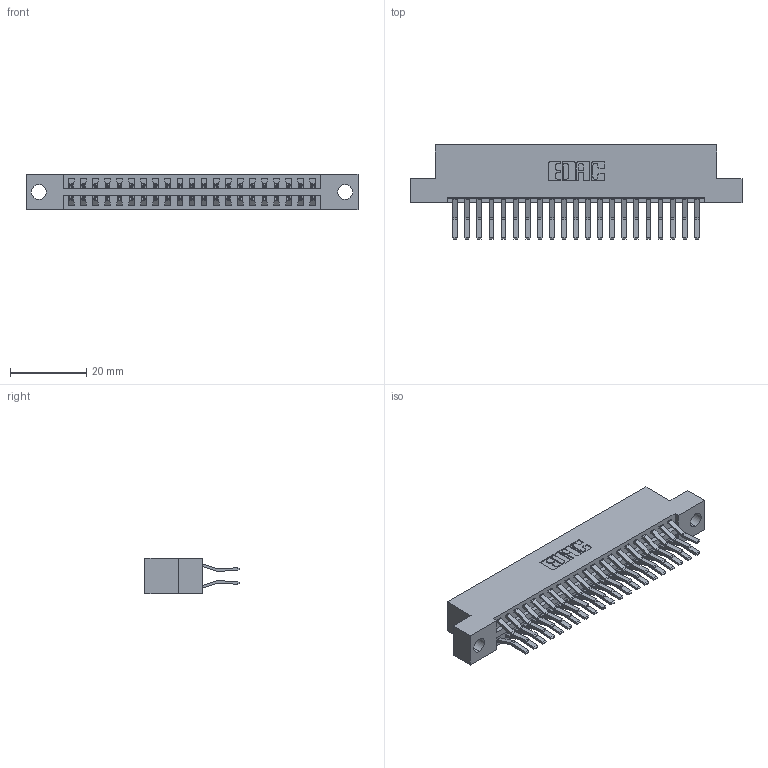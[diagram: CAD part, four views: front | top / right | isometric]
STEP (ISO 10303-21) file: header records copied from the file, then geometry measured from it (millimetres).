
FILE_DESCRIPTION (( 'STEP AP203' ), '1' );
FILE_NAME ('346-042-560-204.STEP', '2022-05-20T05:46:33', ( '' ), ( '' ), 'SwSTEP 2.0', 'SolidWorks 2020', '' );
FILE_SCHEMA (( 'CONFIG_CONTROL_DESIGN' ));
Length unit declared in the file: inch
Products named in the file (3): 346-042-560-204; 346 Part_Flush Mounting Lugs - 0.156 Dia-TH; 345-292-001_560 Tail
Assembly tree (43 placements, depth 2):
  346-042-560-204
    346 Part_Flush Mounting Lugs - 0.156 Dia-TH
    345-292-001_560 Tail  x42
Bounding box: 87.25 x 24.78 x 9.4 mm (x, y, z)
Volume: 8514.1 mm3; surface area: 11955.5 mm2
Topology: 43 solids, 43 shells, 2404 faces, 7127 edges, 4694 vertices
Faces by surface type: plane 1560, cylinder 844
Entity records: 17039 total; most frequent: CARTESIAN_POINT 2842, ORIENTED_EDGE 2774, DIRECTION 2559, EDGE_CURVE 1387, VECTOR 1167, LINE 1167, VERTEX_POINT 922, AXIS2_PLACEMENT_3D 696
